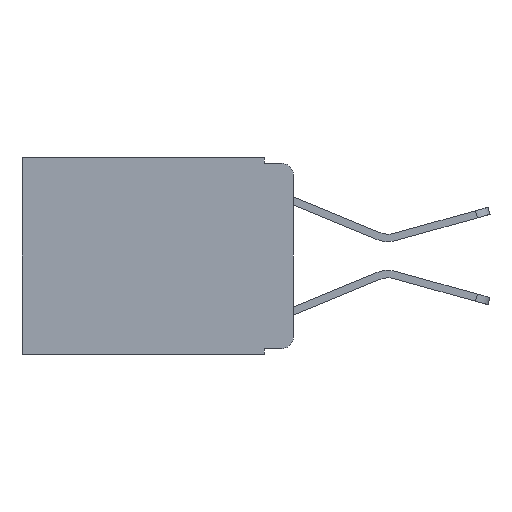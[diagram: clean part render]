
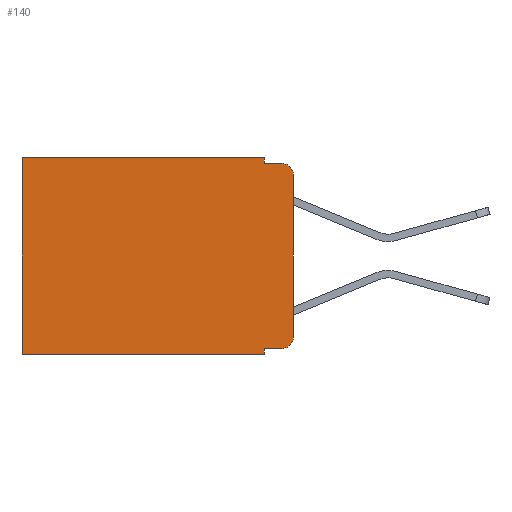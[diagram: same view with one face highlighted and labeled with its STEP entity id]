
A CAD part, left-side view. The second image highlights one B-rep face of the part: STEP entity #140.
In plain terms, the highlighted planar face has unit normal (-1, 0, 0).
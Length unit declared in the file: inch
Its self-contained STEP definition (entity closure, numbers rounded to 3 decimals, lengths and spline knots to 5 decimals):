
#49 = EDGE_LOOP ( 'NONE', ( #2026, #9282, #1600, #6699, #1640, #3852, #5227, #14082, #10637, #2627 ) ) ;
#97 = CARTESIAN_POINT ( 'NONE',  ( 0.298, 0.02, -0.03 ) ) ;
#140 = ADVANCED_FACE ( 'NONE', ( #6964 ), #12121, .F. ) ;
#468 = VECTOR ( 'NONE', #3127, 39.37008 ) ;
#472 = LINE ( 'NONE', #15429, #9843 ) ;
#612 = CARTESIAN_POINT ( 'NONE',  ( 0.298, 0.473, -0.343 ) ) ;
#640 = CARTESIAN_POINT ( 'NONE',  ( 0.298, 0., -0.313 ) ) ;
#915 = LINE ( 'NONE', #8961, #468 ) ;
#931 = DIRECTION ( 'NONE',  ( 0., 0., -1. ) ) ;
#1375 = VECTOR ( 'NONE', #13218, 39.37008 ) ;
#1600 = ORIENTED_EDGE ( 'NONE', *, *, #8519, .F. ) ;
#1640 = ORIENTED_EDGE ( 'NONE', *, *, #9672, .T. ) ;
#1759 = VECTOR ( 'NONE', #931, 39.37008 ) ;
#1780 = AXIS2_PLACEMENT_3D ( 'NONE', #97, #2954, #7263 ) ;
#1790 = LINE ( 'NONE', #8051, #1375 ) ;
#1818 = AXIS2_PLACEMENT_3D ( 'NONE', #10212, #10172, #9687 ) ;
#2021 = VERTEX_POINT ( 'NONE', #14876 ) ;
#2026 = ORIENTED_EDGE ( 'NONE', *, *, #9099, .F. ) ;
#2240 = CARTESIAN_POINT ( 'NONE',  ( 0.298, 0.02, -0.01 ) ) ;
#2540 = CARTESIAN_POINT ( 'NONE',  ( 0.298, 0.051, -0.01 ) ) ;
#2557 = CARTESIAN_POINT ( 'NONE',  ( 0.298, 0., 0. ) ) ;
#2609 = VERTEX_POINT ( 'NONE', #2240 ) ;
#2627 = ORIENTED_EDGE ( 'NONE', *, *, #8401, .T. ) ;
#2631 = CIRCLE ( 'NONE', #1818, 0.02 ) ;
#2954 = DIRECTION ( 'NONE',  ( -1., 0., 0. ) ) ;
#3012 = CARTESIAN_POINT ( 'NONE',  ( 0.298, 0., 0. ) ) ;
#3127 = DIRECTION ( 'NONE',  ( 0., 1., 0. ) ) ;
#3270 = VECTOR ( 'NONE', #3457, 39.37008 ) ;
#3457 = DIRECTION ( 'NONE',  ( 0., -1., 0. ) ) ;
#3852 = ORIENTED_EDGE ( 'NONE', *, *, #8443, .T. ) ;
#5227 = ORIENTED_EDGE ( 'NONE', *, *, #9143, .F. ) ;
#5257 = LINE ( 'NONE', #11958, #8507 ) ;
#5474 = VERTEX_POINT ( 'NONE', #6691 ) ;
#5873 = CARTESIAN_POINT ( 'NONE',  ( 0.298, 0.051, -0.333 ) ) ;
#6042 = LINE ( 'NONE', #8028, #11773 ) ;
#6324 = AXIS2_PLACEMENT_3D ( 'NONE', #3012, #11705, #10895 ) ;
#6691 = CARTESIAN_POINT ( 'NONE',  ( 0.298, 0.473, 0. ) ) ;
#6699 = ORIENTED_EDGE ( 'NONE', *, *, #8446, .F. ) ;
#6964 = FACE_OUTER_BOUND ( 'NONE', #49, .T. ) ;
#7263 = DIRECTION ( 'NONE',  ( 0., 0., -1. ) ) ;
#7346 = LINE ( 'NONE', #10104, #3270 ) ;
#7667 = DIRECTION ( 'NONE',  ( 0., 0., -1. ) ) ;
#7780 = CARTESIAN_POINT ( 'NONE',  ( 0.298, 0.051, 0. ) ) ;
#8028 = CARTESIAN_POINT ( 'NONE',  ( 0.298, 0.051, -0.333 ) ) ;
#8051 = CARTESIAN_POINT ( 'NONE',  ( 0.298, 0.473, 0. ) ) ;
#8109 = LINE ( 'NONE', #7780, #11007 ) ;
#8401 = EDGE_CURVE ( 'NONE', #13888, #8662, #2631, .T. ) ;
#8403 = EDGE_CURVE ( 'NONE', #12198, #13888, #6042, .T. ) ;
#8416 = EDGE_CURVE ( 'NONE', #12198, #14402, #5257, .T. ) ;
#8426 = DIRECTION ( 'NONE',  ( 0., 0., -1. ) ) ;
#8443 = EDGE_CURVE ( 'NONE', #5474, #14916, #1790, .T. ) ;
#8446 = EDGE_CURVE ( 'NONE', #9549, #15110, #8109, .T. ) ;
#8468 = EDGE_CURVE ( 'NONE', #2021, #2609, #14190, .T. ) ;
#8507 = VECTOR ( 'NONE', #8426, 39.37008 ) ;
#8519 = EDGE_CURVE ( 'NONE', #15110, #2609, #7346, .T. ) ;
#8662 = VERTEX_POINT ( 'NONE', #640 ) ;
#8860 = LINE ( 'NONE', #2557, #1759 ) ;
#8961 = CARTESIAN_POINT ( 'NONE',  ( 0.298, 0., -0.343 ) ) ;
#9099 = EDGE_CURVE ( 'NONE', #2021, #8662, #8860, .T. ) ;
#9143 = EDGE_CURVE ( 'NONE', #14402, #14916, #915, .T. ) ;
#9282 = ORIENTED_EDGE ( 'NONE', *, *, #8468, .T. ) ;
#9549 = VERTEX_POINT ( 'NONE', #15180 ) ;
#9672 = EDGE_CURVE ( 'NONE', #9549, #5474, #472, .T. ) ;
#9687 = DIRECTION ( 'NONE',  ( 0., 0., -1. ) ) ;
#9843 = VECTOR ( 'NONE', #14307, 39.37008 ) ;
#10104 = CARTESIAN_POINT ( 'NONE',  ( 0.298, 0.051, -0.01 ) ) ;
#10172 = DIRECTION ( 'NONE',  ( -1., 0., 0. ) ) ;
#10212 = CARTESIAN_POINT ( 'NONE',  ( 0.298, 0.02, -0.313 ) ) ;
#10281 = DIRECTION ( 'NONE',  ( 0., -1., 0. ) ) ;
#10637 = ORIENTED_EDGE ( 'NONE', *, *, #8403, .T. ) ;
#10895 = DIRECTION ( 'NONE',  ( 0., 0., -1. ) ) ;
#11007 = VECTOR ( 'NONE', #7667, 39.37008 ) ;
#11705 = DIRECTION ( 'NONE',  ( 1., 0., 0. ) ) ;
#11773 = VECTOR ( 'NONE', #10281, 39.37008 ) ;
#11958 = CARTESIAN_POINT ( 'NONE',  ( 0.298, 0.051, 0. ) ) ;
#12121 = PLANE ( 'NONE',  #6324 ) ;
#12198 = VERTEX_POINT ( 'NONE', #5873 ) ;
#13218 = DIRECTION ( 'NONE',  ( 0., 0., -1. ) ) ;
#13888 = VERTEX_POINT ( 'NONE', #14789 ) ;
#13955 = CARTESIAN_POINT ( 'NONE',  ( 0.298, 0.051, -0.343 ) ) ;
#14082 = ORIENTED_EDGE ( 'NONE', *, *, #8416, .F. ) ;
#14190 = CIRCLE ( 'NONE', #1780, 0.02 ) ;
#14307 = DIRECTION ( 'NONE',  ( 0., 1., 0. ) ) ;
#14402 = VERTEX_POINT ( 'NONE', #13955 ) ;
#14789 = CARTESIAN_POINT ( 'NONE',  ( 0.298, 0.02, -0.333 ) ) ;
#14876 = CARTESIAN_POINT ( 'NONE',  ( 0.298, 0., -0.03 ) ) ;
#14916 = VERTEX_POINT ( 'NONE', #612 ) ;
#15110 = VERTEX_POINT ( 'NONE', #2540 ) ;
#15180 = CARTESIAN_POINT ( 'NONE',  ( 0.298, 0.051, 0. ) ) ;
#15429 = CARTESIAN_POINT ( 'NONE',  ( 0.298, 0., 0. ) ) ;
